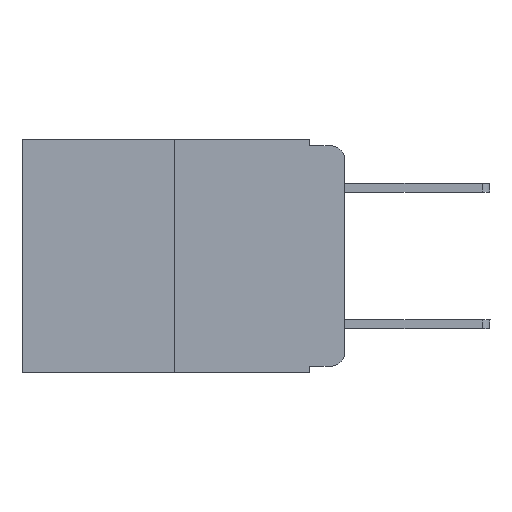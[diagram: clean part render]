
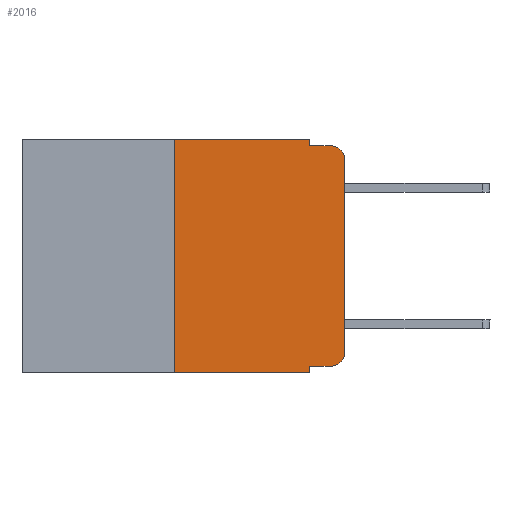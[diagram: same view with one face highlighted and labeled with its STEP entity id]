
A CAD part, left-side view. The second image highlights one B-rep face of the part: STEP entity #2016.
In plain terms, the highlighted planar face has unit normal (-1, 0, 0).
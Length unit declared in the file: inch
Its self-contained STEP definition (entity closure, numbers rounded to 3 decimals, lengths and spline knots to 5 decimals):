
#6 = ORIENTED_EDGE ( 'NONE', *, *, #3581, .T. ) ;
#344 = EDGE_CURVE ( 'NONE', #7582, #4872, #2667, .T. ) ;
#962 = ORIENTED_EDGE ( 'NONE', *, *, #4498, .F. ) ;
#1129 = CARTESIAN_POINT ( 'NONE',  ( 0., 0.051, 0. ) ) ;
#1349 = CARTESIAN_POINT ( 'NONE',  ( 0., 0., -0.03 ) ) ;
#1427 = DIRECTION ( 'NONE',  ( 0., -1., 0. ) ) ;
#1714 = DIRECTION ( 'NONE',  ( 1., 0., 0. ) ) ;
#1763 = DIRECTION ( 'NONE',  ( 0., 0., 1. ) ) ;
#1880 = LINE ( 'NONE', #1129, #4394 ) ;
#2016 = ADVANCED_FACE ( 'NONE', ( #3296 ), #9041, .F. ) ;
#2084 = VERTEX_POINT ( 'NONE', #8185 ) ;
#2087 = CARTESIAN_POINT ( 'NONE',  ( 0., 0.473, 0. ) ) ;
#2159 = CARTESIAN_POINT ( 'NONE',  ( 0., 0.051, -0.343 ) ) ;
#2222 = VECTOR ( 'NONE', #9609, 39.37008 ) ;
#2467 = EDGE_CURVE ( 'NONE', #2804, #10097, #7320, .T. ) ;
#2590 = CARTESIAN_POINT ( 'NONE',  ( 0., 0.25, -0.343 ) ) ;
#2667 = LINE ( 'NONE', #2087, #10218 ) ;
#2697 = AXIS2_PLACEMENT_3D ( 'NONE', #4538, #3740, #8627 ) ;
#2708 = LINE ( 'NONE', #8510, #2818 ) ;
#2716 = LINE ( 'NONE', #2819, #10358 ) ;
#2804 = VERTEX_POINT ( 'NONE', #6042 ) ;
#2818 = VECTOR ( 'NONE', #5963, 39.37008 ) ;
#2819 = CARTESIAN_POINT ( 'NONE',  ( 0., 0.051, 0. ) ) ;
#2850 = VECTOR ( 'NONE', #7397, 39.37008 ) ;
#2928 = EDGE_CURVE ( 'NONE', #2084, #6058, #6552, .T. ) ;
#2979 = EDGE_CURVE ( 'NONE', #3919, #7582, #3409, .T. ) ;
#3070 = EDGE_CURVE ( 'NONE', #2084, #5044, #2716, .T. ) ;
#3285 = ORIENTED_EDGE ( 'NONE', *, *, #2928, .T. ) ;
#3296 = FACE_OUTER_BOUND ( 'NONE', #7238, .T. ) ;
#3395 = DIRECTION ( 'NONE',  ( -1., 0., 0. ) ) ;
#3409 = LINE ( 'NONE', #9046, #6947 ) ;
#3445 = ORIENTED_EDGE ( 'NONE', *, *, #3070, .F. ) ;
#3556 = CARTESIAN_POINT ( 'NONE',  ( 0., 0.02, -0.313 ) ) ;
#3581 = EDGE_CURVE ( 'NONE', #6058, #2804, #8060, .T. ) ;
#3688 = ORIENTED_EDGE ( 'NONE', *, *, #7962, .T. ) ;
#3740 = DIRECTION ( 'NONE',  ( -1., 0., 0. ) ) ;
#3919 = VERTEX_POINT ( 'NONE', #2590 ) ;
#3935 = ORIENTED_EDGE ( 'NONE', *, *, #2979, .F. ) ;
#4278 = ORIENTED_EDGE ( 'NONE', *, *, #7329, .T. ) ;
#4381 = CARTESIAN_POINT ( 'NONE',  ( 0., 0.02, -0.01 ) ) ;
#4394 = VECTOR ( 'NONE', #6764, 39.37008 ) ;
#4498 = EDGE_CURVE ( 'NONE', #5327, #9932, #2708, .T. ) ;
#4538 = CARTESIAN_POINT ( 'NONE',  ( 0., 0.02, -0.03 ) ) ;
#4668 = CARTESIAN_POINT ( 'NONE',  ( 0., 0.02, -0.333 ) ) ;
#4872 = VERTEX_POINT ( 'NONE', #5797 ) ;
#4954 = CARTESIAN_POINT ( 'NONE',  ( 0., 0.473, 0. ) ) ;
#5044 = VERTEX_POINT ( 'NONE', #2159 ) ;
#5059 = DIRECTION ( 'NONE',  ( 0., 0., -1. ) ) ;
#5082 = VECTOR ( 'NONE', #1427, 39.37008 ) ;
#5327 = VERTEX_POINT ( 'NONE', #6623 ) ;
#5331 = DIRECTION ( 'NONE',  ( 0., -1., 0. ) ) ;
#5741 = LINE ( 'NONE', #6326, #5082 ) ;
#5797 = CARTESIAN_POINT ( 'NONE',  ( 0., 0.051, 0. ) ) ;
#5963 = DIRECTION ( 'NONE',  ( 0., -1., 0. ) ) ;
#6042 = CARTESIAN_POINT ( 'NONE',  ( 0., 0., -0.313 ) ) ;
#6047 = ORIENTED_EDGE ( 'NONE', *, *, #344, .F. ) ;
#6058 = VERTEX_POINT ( 'NONE', #4668 ) ;
#6326 = CARTESIAN_POINT ( 'NONE',  ( 0., 0.473, -0.343 ) ) ;
#6552 = LINE ( 'NONE', #9899, #2850 ) ;
#6623 = CARTESIAN_POINT ( 'NONE',  ( 0., 0.051, -0.01 ) ) ;
#6764 = DIRECTION ( 'NONE',  ( 0., 0., -1. ) ) ;
#6947 = VECTOR ( 'NONE', #1763, 39.37008 ) ;
#7078 = ORIENTED_EDGE ( 'NONE', *, *, #7186, .F. ) ;
#7103 = CIRCLE ( 'NONE', #2697, 0.02 ) ;
#7186 = EDGE_CURVE ( 'NONE', #4872, #5327, #1880, .T. ) ;
#7238 = EDGE_LOOP ( 'NONE', ( #10455, #4278, #962, #7078, #6047, #3935, #3688, #3445, #3285, #6 ) ) ;
#7320 = LINE ( 'NONE', #8174, #2222 ) ;
#7329 = EDGE_CURVE ( 'NONE', #10097, #9932, #7103, .T. ) ;
#7397 = DIRECTION ( 'NONE',  ( 0., -1., 0. ) ) ;
#7582 = VERTEX_POINT ( 'NONE', #9152 ) ;
#7727 = AXIS2_PLACEMENT_3D ( 'NONE', #3556, #3395, #10053 ) ;
#7962 = EDGE_CURVE ( 'NONE', #3919, #5044, #5741, .T. ) ;
#8060 = CIRCLE ( 'NONE', #7727, 0.02 ) ;
#8174 = CARTESIAN_POINT ( 'NONE',  ( 0., 0., 0. ) ) ;
#8185 = CARTESIAN_POINT ( 'NONE',  ( 0., 0.051, -0.333 ) ) ;
#8510 = CARTESIAN_POINT ( 'NONE',  ( 0., 0.051, -0.01 ) ) ;
#8627 = DIRECTION ( 'NONE',  ( 0., 0., -1. ) ) ;
#9041 = PLANE ( 'NONE',  #9365 ) ;
#9046 = CARTESIAN_POINT ( 'NONE',  ( 0., 0.25, 0. ) ) ;
#9091 = DIRECTION ( 'NONE',  ( 0., 0., -1. ) ) ;
#9152 = CARTESIAN_POINT ( 'NONE',  ( 0., 0.25, 0. ) ) ;
#9365 = AXIS2_PLACEMENT_3D ( 'NONE', #4954, #1714, #9091 ) ;
#9609 = DIRECTION ( 'NONE',  ( 0., 0., 1. ) ) ;
#9899 = CARTESIAN_POINT ( 'NONE',  ( 0., 0.051, -0.333 ) ) ;
#9932 = VERTEX_POINT ( 'NONE', #4381 ) ;
#10053 = DIRECTION ( 'NONE',  ( 0., 0., -1. ) ) ;
#10097 = VERTEX_POINT ( 'NONE', #1349 ) ;
#10218 = VECTOR ( 'NONE', #5331, 39.37008 ) ;
#10358 = VECTOR ( 'NONE', #5059, 39.37008 ) ;
#10455 = ORIENTED_EDGE ( 'NONE', *, *, #2467, .T. ) ;
